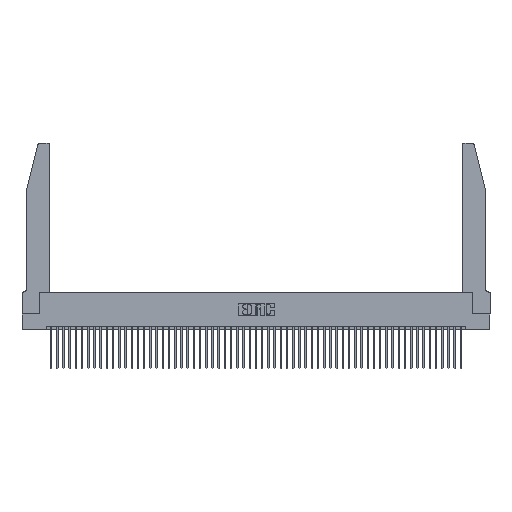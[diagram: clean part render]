
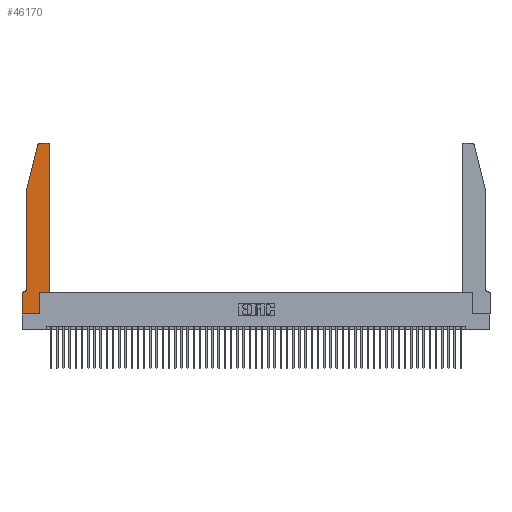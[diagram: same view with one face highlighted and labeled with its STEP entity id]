
A CAD part, top view. The second image highlights one B-rep face of the part: STEP entity #46170.
In plain terms, the highlighted planar face has unit normal (0, 0, 1).
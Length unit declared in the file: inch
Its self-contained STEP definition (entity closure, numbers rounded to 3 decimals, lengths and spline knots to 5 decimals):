
#510 = CARTESIAN_POINT ( 'NONE',  ( 0., 0., 0.37 ) ) ;
#711 = CARTESIAN_POINT ( 'NONE',  ( 0.4205, 2.72, 0.37 ) ) ;
#945 = AXIS2_PLACEMENT_3D ( 'NONE', #13886, #22103, #34327 ) ;
#1000 = LINE ( 'NONE', #11362, #43425 ) ;
#2045 = CARTESIAN_POINT ( 'NONE',  ( 0.284, 2.72, 0.37 ) ) ;
#2267 = EDGE_CURVE ( 'NONE', #11865, #53175, #23957, .T. ) ;
#2500 = EDGE_CURVE ( 'NONE', #27809, #11865, #53224, .T. ) ;
#4160 = LINE ( 'NONE', #31431, #37815 ) ;
#4358 = DIRECTION ( 'NONE',  ( 1., 0., 0. ) ) ;
#4811 = ORIENTED_EDGE ( 'NONE', *, *, #6293, .T. ) ;
#5288 = ORIENTED_EDGE ( 'NONE', *, *, #47582, .T. ) ;
#5380 = LINE ( 'NONE', #14317, #48516 ) ;
#6293 = EDGE_CURVE ( 'NONE', #53175, #52478, #11605, .T. ) ;
#6804 = CIRCLE ( 'NONE', #49895, 0.03 ) ;
#8449 = EDGE_CURVE ( 'NONE', #52478, #44650, #47388, .T. ) ;
#8734 = DIRECTION ( 'NONE',  ( -1., 0., 0. ) ) ;
#9276 = ORIENTED_EDGE ( 'NONE', *, *, #2500, .T. ) ;
#9658 = VECTOR ( 'NONE', #51237, 39.37008 ) ;
#10240 = EDGE_CURVE ( 'NONE', #37798, #34402, #32124, .T. ) ;
#10531 = CARTESIAN_POINT ( 'NONE',  ( 0.25487, 2.72718, 0.37 ) ) ;
#11362 = CARTESIAN_POINT ( 'NONE',  ( 0.0755, 2., 0.37 ) ) ;
#11605 = LINE ( 'NONE', #510, #9658 ) ;
#11865 = VERTEX_POINT ( 'NONE', #28739 ) ;
#12733 = FACE_OUTER_BOUND ( 'NONE', #26527, .T. ) ;
#13886 = CARTESIAN_POINT ( 'NONE',  ( 0., 0.35, 0.37 ) ) ;
#13994 = ORIENTED_EDGE ( 'NONE', *, *, #46744, .T. ) ;
#14317 = CARTESIAN_POINT ( 'NONE',  ( 0.4505, 0.35, 0.37 ) ) ;
#18302 = DIRECTION ( 'NONE',  ( 0., 1., 0. ) ) ;
#18736 = CARTESIAN_POINT ( 'NONE',  ( 0.0755, 2., 0.37 ) ) ;
#18748 = CARTESIAN_POINT ( 'NONE',  ( 0., 0., 0.37 ) ) ;
#20695 = LINE ( 'NONE', #44222, #45509 ) ;
#21331 = CARTESIAN_POINT ( 'NONE',  ( 0., 0., 0.37 ) ) ;
#21635 = VECTOR ( 'NONE', #30413, 39.37008 ) ;
#22103 = DIRECTION ( 'NONE',  ( 0., 0., 1. ) ) ;
#22421 = DIRECTION ( 'NONE',  ( 0., 0., -1. ) ) ;
#23317 = ORIENTED_EDGE ( 'NONE', *, *, #8449, .T. ) ;
#23957 = LINE ( 'NONE', #37729, #29823 ) ;
#25880 = VERTEX_POINT ( 'NONE', #53872 ) ;
#26099 = DIRECTION ( 'NONE',  ( 1., 0., 0. ) ) ;
#26527 = EDGE_LOOP ( 'NONE', ( #36679, #38120, #37960, #40098, #9276, #29995, #4811, #23317, #29377, #42870, #5288, #13994 ) ) ;
#27298 = EDGE_CURVE ( 'NONE', #39961, #34059, #20695, .T. ) ;
#27809 = VERTEX_POINT ( 'NONE', #46709 ) ;
#28186 = LINE ( 'NONE', #53615, #49070 ) ;
#28739 = CARTESIAN_POINT ( 'NONE',  ( 0.0055, 0.35, 0.37 ) ) ;
#29048 = CIRCLE ( 'NONE', #48577, 0.03 ) ;
#29342 = CARTESIAN_POINT ( 'NONE',  ( 0.284, 2.75, 0.37 ) ) ;
#29371 = DIRECTION ( 'NONE',  ( 0., 0., 1. ) ) ;
#29377 = ORIENTED_EDGE ( 'NONE', *, *, #32903, .T. ) ;
#29823 = VECTOR ( 'NONE', #8734, 39.37008 ) ;
#29995 = ORIENTED_EDGE ( 'NONE', *, *, #2267, .T. ) ;
#30413 = DIRECTION ( 'NONE',  ( 1., 0., 0. ) ) ;
#31431 = CARTESIAN_POINT ( 'NONE',  ( 0.2865, 0.35, 0.37 ) ) ;
#32124 = LINE ( 'NONE', #51739, #21635 ) ;
#32719 = AXIS2_PLACEMENT_3D ( 'NONE', #43967, #22421, #34819 ) ;
#32903 = EDGE_CURVE ( 'NONE', #44650, #37798, #4160, .T. ) ;
#33234 = DIRECTION ( 'NONE',  ( -1., 0., 0. ) ) ;
#33810 = VERTEX_POINT ( 'NONE', #29342 ) ;
#33963 = CARTESIAN_POINT ( 'NONE',  ( 0.2865, 0.35, 0.37 ) ) ;
#34059 = VERTEX_POINT ( 'NONE', #18736 ) ;
#34327 = DIRECTION ( 'NONE',  ( 1., 0., 0. ) ) ;
#34402 = VERTEX_POINT ( 'NONE', #45871 ) ;
#34691 = DIRECTION ( 'NONE',  ( 0., 0., 1. ) ) ;
#34819 = DIRECTION ( 'NONE',  ( -1., 0., 0. ) ) ;
#36679 = ORIENTED_EDGE ( 'NONE', *, *, #40934, .T. ) ;
#37729 = CARTESIAN_POINT ( 'NONE',  ( 0.0755, 0.35, 0.37 ) ) ;
#37798 = VERTEX_POINT ( 'NONE', #33963 ) ;
#37815 = VECTOR ( 'NONE', #18302, 39.37008 ) ;
#37883 = EDGE_CURVE ( 'NONE', #33810, #39961, #29048, .T. ) ;
#37960 = ORIENTED_EDGE ( 'NONE', *, *, #27298, .T. ) ;
#38120 = ORIENTED_EDGE ( 'NONE', *, *, #37883, .T. ) ;
#39287 = DIRECTION ( 'NONE',  ( 1., 0., 0. ) ) ;
#39961 = VERTEX_POINT ( 'NONE', #10531 ) ;
#40098 = ORIENTED_EDGE ( 'NONE', *, *, #45790, .T. ) ;
#40934 = EDGE_CURVE ( 'NONE', #49365, #33810, #28186, .T. ) ;
#41494 = VECTOR ( 'NONE', #26099, 39.37008 ) ;
#42870 = ORIENTED_EDGE ( 'NONE', *, *, #10240, .T. ) ;
#43097 = CARTESIAN_POINT ( 'NONE',  ( 0.4205, 2.75, 0.37 ) ) ;
#43425 = VECTOR ( 'NONE', #45134, 39.37008 ) ;
#43967 = CARTESIAN_POINT ( 'NONE',  ( 0.0055, 0.42, 0.37 ) ) ;
#44222 = CARTESIAN_POINT ( 'NONE',  ( 0.0755, 2., 0.37 ) ) ;
#44650 = VERTEX_POINT ( 'NONE', #52619 ) ;
#44759 = CARTESIAN_POINT ( 'NONE',  ( 0., 0.35, 0.37 ) ) ;
#45134 = DIRECTION ( 'NONE',  ( 0., -1., 0. ) ) ;
#45509 = VECTOR ( 'NONE', #48058, 39.37008 ) ;
#45790 = EDGE_CURVE ( 'NONE', #34059, #27809, #1000, .T. ) ;
#45871 = CARTESIAN_POINT ( 'NONE',  ( 0.4505, 0.35, 0.37 ) ) ;
#46170 = ADVANCED_FACE ( 'NONE', ( #12733 ), #46757, .T. ) ;
#46709 = CARTESIAN_POINT ( 'NONE',  ( 0.0755, 0.42, 0.37 ) ) ;
#46744 = EDGE_CURVE ( 'NONE', #25880, #49365, #6804, .T. ) ;
#46757 = PLANE ( 'NONE',  #945 ) ;
#47371 = DIRECTION ( 'NONE',  ( 0., 1., 0. ) ) ;
#47388 = LINE ( 'NONE', #21331, #41494 ) ;
#47582 = EDGE_CURVE ( 'NONE', #34402, #25880, #5380, .T. ) ;
#48058 = DIRECTION ( 'NONE',  ( -0.239, -0.971, 0. ) ) ;
#48516 = VECTOR ( 'NONE', #47371, 39.37008 ) ;
#48577 = AXIS2_PLACEMENT_3D ( 'NONE', #2045, #34691, #39287 ) ;
#49070 = VECTOR ( 'NONE', #33234, 39.37008 ) ;
#49365 = VERTEX_POINT ( 'NONE', #43097 ) ;
#49895 = AXIS2_PLACEMENT_3D ( 'NONE', #711, #29371, #4358 ) ;
#51237 = DIRECTION ( 'NONE',  ( 0., -1., 0. ) ) ;
#51739 = CARTESIAN_POINT ( 'NONE',  ( 0.4505, 0.35, 0.37 ) ) ;
#52478 = VERTEX_POINT ( 'NONE', #18748 ) ;
#52619 = CARTESIAN_POINT ( 'NONE',  ( 0.2865, 0., 0.37 ) ) ;
#53175 = VERTEX_POINT ( 'NONE', #44759 ) ;
#53224 = CIRCLE ( 'NONE', #32719, 0.07 ) ;
#53615 = CARTESIAN_POINT ( 'NONE',  ( 0.2605, 2.75, 0.37 ) ) ;
#53872 = CARTESIAN_POINT ( 'NONE',  ( 0.4505, 2.72, 0.37 ) ) ;
